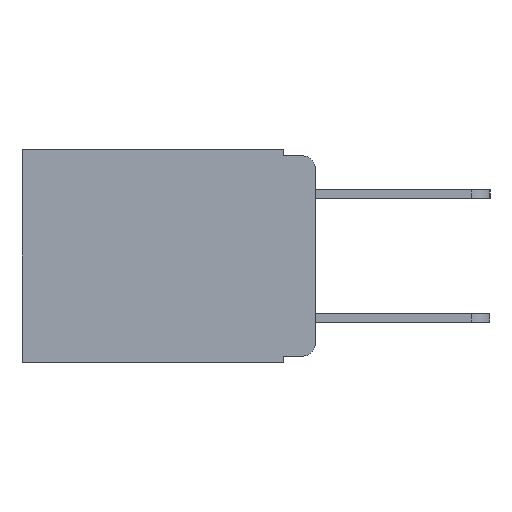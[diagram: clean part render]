
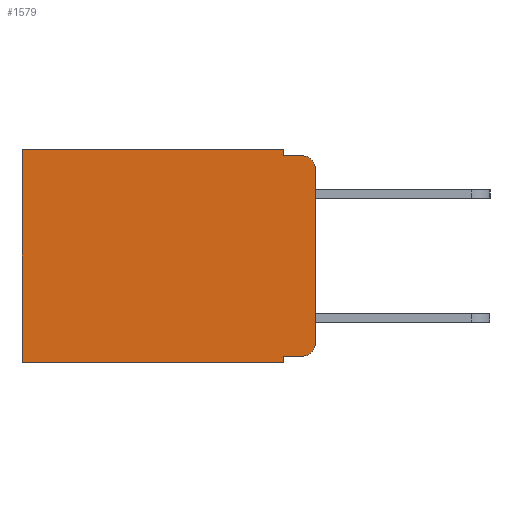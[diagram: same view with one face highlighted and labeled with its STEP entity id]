
A CAD part, left-side view. The second image highlights one B-rep face of the part: STEP entity #1579.
In plain terms, the highlighted planar face has unit normal (-1, 0, 0).
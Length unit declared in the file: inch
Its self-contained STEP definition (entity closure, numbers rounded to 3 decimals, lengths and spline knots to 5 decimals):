
#114 = ORIENTED_EDGE ( 'NONE', *, *, #8239, .F. ) ;
#143 = CARTESIAN_POINT ( 'NONE',  ( 0.298, 0.473, -0.343 ) ) ;
#331 = EDGE_CURVE ( 'NONE', #3140, #5931, #8701, .T. ) ;
#403 = ORIENTED_EDGE ( 'NONE', *, *, #8877, .F. ) ;
#494 = CARTESIAN_POINT ( 'NONE',  ( 0.298, 0.051, -0.333 ) ) ;
#712 = DIRECTION ( 'NONE',  ( 0., 0., -1. ) ) ;
#721 = CARTESIAN_POINT ( 'NONE',  ( 0.298, 0.051, 0. ) ) ;
#839 = EDGE_CURVE ( 'NONE', #5574, #8420, #1862, .T. ) ;
#968 = CARTESIAN_POINT ( 'NONE',  ( 0.298, 0.02, -0.03 ) ) ;
#987 = ORIENTED_EDGE ( 'NONE', *, *, #331, .T. ) ;
#988 = CARTESIAN_POINT ( 'NONE',  ( 0.298, 0.473, 0. ) ) ;
#1103 = CARTESIAN_POINT ( 'NONE',  ( 0.298, 0.051, 0. ) ) ;
#1109 = DIRECTION ( 'NONE',  ( 0., -1., 0. ) ) ;
#1278 = LINE ( 'NONE', #1103, #9363 ) ;
#1383 = EDGE_CURVE ( 'NONE', #2210, #2756, #1278, .T. ) ;
#1438 = CARTESIAN_POINT ( 'NONE',  ( 0.298, 0.473, 0. ) ) ;
#1490 = VERTEX_POINT ( 'NONE', #6750 ) ;
#1546 = DIRECTION ( 'NONE',  ( 0., 0., -1. ) ) ;
#1566 = CARTESIAN_POINT ( 'NONE',  ( 0.298, 0.051, -0.343 ) ) ;
#1579 = ADVANCED_FACE ( 'NONE', ( #7695 ), #5800, .F. ) ;
#1581 = ORIENTED_EDGE ( 'NONE', *, *, #1383, .F. ) ;
#1613 = DIRECTION ( 'NONE',  ( 0., 0., -1. ) ) ;
#1652 = EDGE_CURVE ( 'NONE', #2756, #5931, #6484, .T. ) ;
#1762 = CARTESIAN_POINT ( 'NONE',  ( 0.298, 0.051, 0. ) ) ;
#1832 = ORIENTED_EDGE ( 'NONE', *, *, #4483, .T. ) ;
#1862 = LINE ( 'NONE', #1438, #9836 ) ;
#1863 = LINE ( 'NONE', #5473, #8368 ) ;
#1924 = ORIENTED_EDGE ( 'NONE', *, *, #1652, .F. ) ;
#2210 = VERTEX_POINT ( 'NONE', #1762 ) ;
#2751 = VERTEX_POINT ( 'NONE', #1566 ) ;
#2756 = VERTEX_POINT ( 'NONE', #9513 ) ;
#2810 = ORIENTED_EDGE ( 'NONE', *, *, #839, .T. ) ;
#3140 = VERTEX_POINT ( 'NONE', #4360 ) ;
#3158 = VERTEX_POINT ( 'NONE', #494 ) ;
#3215 = DIRECTION ( 'NONE',  ( -1., 0., 0. ) ) ;
#3316 = DIRECTION ( 'NONE',  ( 0., 0., -1. ) ) ;
#3482 = DIRECTION ( 'NONE',  ( 0., 0., -1. ) ) ;
#3941 = AXIS2_PLACEMENT_3D ( 'NONE', #10623, #6153, #712 ) ;
#3992 = DIRECTION ( 'NONE',  ( 1., 0., 0. ) ) ;
#4148 = VECTOR ( 'NONE', #6100, 39.37008 ) ;
#4272 = VECTOR ( 'NONE', #1613, 39.37008 ) ;
#4357 = LINE ( 'NONE', #9061, #6681 ) ;
#4360 = CARTESIAN_POINT ( 'NONE',  ( 0.298, 0., -0.03 ) ) ;
#4483 = EDGE_CURVE ( 'NONE', #2210, #5574, #4357, .T. ) ;
#5106 = CIRCLE ( 'NONE', #3941, 0.02 ) ;
#5473 = CARTESIAN_POINT ( 'NONE',  ( 0.298, 0., -0.343 ) ) ;
#5574 = VERTEX_POINT ( 'NONE', #988 ) ;
#5694 = LINE ( 'NONE', #9022, #9506 ) ;
#5800 = PLANE ( 'NONE',  #5835 ) ;
#5835 = AXIS2_PLACEMENT_3D ( 'NONE', #9573, #3992, #8830 ) ;
#5931 = VERTEX_POINT ( 'NONE', #6427 ) ;
#5976 = DIRECTION ( 'NONE',  ( 0., 0., -1. ) ) ;
#5998 = ORIENTED_EDGE ( 'NONE', *, *, #7266, .T. ) ;
#6100 = DIRECTION ( 'NONE',  ( 0., -1., 0. ) ) ;
#6153 = DIRECTION ( 'NONE',  ( -1., 0., 0. ) ) ;
#6379 = VECTOR ( 'NONE', #5976, 39.37008 ) ;
#6427 = CARTESIAN_POINT ( 'NONE',  ( 0.298, 0.02, -0.01 ) ) ;
#6484 = LINE ( 'NONE', #6957, #4148 ) ;
#6519 = ORIENTED_EDGE ( 'NONE', *, *, #6790, .F. ) ;
#6681 = VECTOR ( 'NONE', #8901, 39.37008 ) ;
#6750 = CARTESIAN_POINT ( 'NONE',  ( 0.298, 0., -0.313 ) ) ;
#6790 = EDGE_CURVE ( 'NONE', #3140, #1490, #8383, .T. ) ;
#6858 = CARTESIAN_POINT ( 'NONE',  ( 0.298, 0., 0. ) ) ;
#6957 = CARTESIAN_POINT ( 'NONE',  ( 0.298, 0.051, -0.01 ) ) ;
#7266 = EDGE_CURVE ( 'NONE', #3158, #10584, #5694, .T. ) ;
#7695 = FACE_OUTER_BOUND ( 'NONE', #8643, .T. ) ;
#8239 = EDGE_CURVE ( 'NONE', #2751, #8420, #1863, .T. ) ;
#8368 = VECTOR ( 'NONE', #10064, 39.37008 ) ;
#8383 = LINE ( 'NONE', #6858, #6379 ) ;
#8420 = VERTEX_POINT ( 'NONE', #143 ) ;
#8643 = EDGE_LOOP ( 'NONE', ( #6519, #987, #1924, #1581, #1832, #2810, #114, #403, #5998, #10116 ) ) ;
#8701 = CIRCLE ( 'NONE', #10819, 0.02 ) ;
#8811 = CARTESIAN_POINT ( 'NONE',  ( 0.298, 0.02, -0.333 ) ) ;
#8830 = DIRECTION ( 'NONE',  ( 0., 0., -1. ) ) ;
#8877 = EDGE_CURVE ( 'NONE', #3158, #2751, #10313, .T. ) ;
#8901 = DIRECTION ( 'NONE',  ( 0., 1., 0. ) ) ;
#9022 = CARTESIAN_POINT ( 'NONE',  ( 0.298, 0.051, -0.333 ) ) ;
#9061 = CARTESIAN_POINT ( 'NONE',  ( 0.298, 0., 0. ) ) ;
#9363 = VECTOR ( 'NONE', #3316, 39.37008 ) ;
#9506 = VECTOR ( 'NONE', #1109, 39.37008 ) ;
#9513 = CARTESIAN_POINT ( 'NONE',  ( 0.298, 0.051, -0.01 ) ) ;
#9573 = CARTESIAN_POINT ( 'NONE',  ( 0.298, 0., 0. ) ) ;
#9693 = EDGE_CURVE ( 'NONE', #10584, #1490, #5106, .T. ) ;
#9836 = VECTOR ( 'NONE', #1546, 39.37008 ) ;
#10064 = DIRECTION ( 'NONE',  ( 0., 1., 0. ) ) ;
#10116 = ORIENTED_EDGE ( 'NONE', *, *, #9693, .T. ) ;
#10313 = LINE ( 'NONE', #721, #4272 ) ;
#10584 = VERTEX_POINT ( 'NONE', #8811 ) ;
#10623 = CARTESIAN_POINT ( 'NONE',  ( 0.298, 0.02, -0.313 ) ) ;
#10819 = AXIS2_PLACEMENT_3D ( 'NONE', #968, #3215, #3482 ) ;
